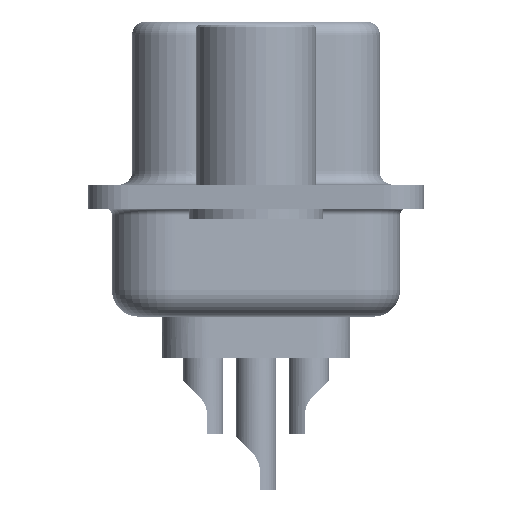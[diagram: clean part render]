
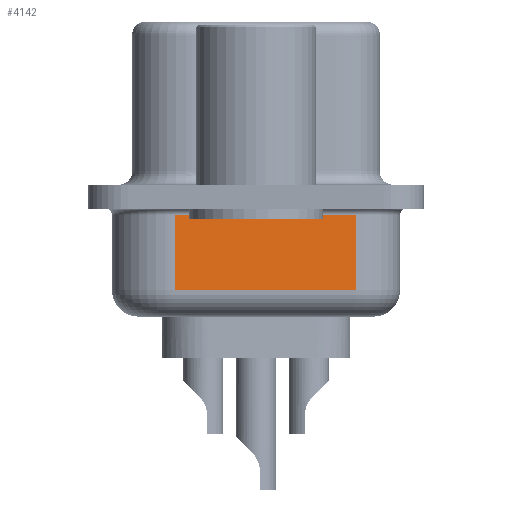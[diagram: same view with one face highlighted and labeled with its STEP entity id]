
A CAD part, left-side view. The second image highlights one B-rep face of the part: STEP entity #4142.
In plain terms, the highlighted planar face has unit normal (-0.985, -0.174, 0).
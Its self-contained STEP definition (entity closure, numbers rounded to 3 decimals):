
#44 = ORIENTED_EDGE ( 'NONE', *, *, #11190, .T. ) ;
#349 = EDGE_LOOP ( 'NONE', ( #19495, #44, #11749, #1574 ) ) ;
#593 = DIRECTION ( 'NONE',  ( 0., 0., 1. ) ) ;
#1041 = LINE ( 'NONE', #5209, #23317 ) ;
#1204 = CARTESIAN_POINT ( 'NONE',  ( 4.199, -3.747, -0.7 ) ) ;
#1379 = LINE ( 'NONE', #17974, #13663 ) ;
#1574 = ORIENTED_EDGE ( 'NONE', *, *, #20124, .T. ) ;
#1625 = FACE_OUTER_BOUND ( 'NONE', #349, .T. ) ;
#1770 = CARTESIAN_POINT ( 'NONE',  ( 3., 3.053, -4.5 ) ) ;
#2224 = VERTEX_POINT ( 'NONE', #1204 ) ;
#2486 = VECTOR ( 'NONE', #16854, 1000. ) ;
#3147 = CARTESIAN_POINT ( 'NONE',  ( 3., 3.053, -3.5 ) ) ;
#4142 = ADVANCED_FACE ( 'NONE', ( #1625 ), #8680, .F. ) ;
#4247 = AXIS2_PLACEMENT_3D ( 'NONE', #1770, #8997, #6689 ) ;
#5209 = CARTESIAN_POINT ( 'NONE',  ( 3., 3.053, -4.5 ) ) ;
#6689 = DIRECTION ( 'NONE',  ( -0.174, 0.985, 0. ) ) ;
#7465 = LINE ( 'NONE', #7762, #2486 ) ;
#7762 = CARTESIAN_POINT ( 'NONE',  ( 4.199, -3.747, -4.5 ) ) ;
#8680 = PLANE ( 'NONE',  #4247 ) ;
#8728 = CARTESIAN_POINT ( 'NONE',  ( 3., 3.053, -0.7 ) ) ;
#8997 = DIRECTION ( 'NONE',  ( 0.985, 0.174, 0. ) ) ;
#11190 = EDGE_CURVE ( 'NONE', #14868, #15572, #1379, .T. ) ;
#11749 = ORIENTED_EDGE ( 'NONE', *, *, #14856, .T. ) ;
#12073 = CARTESIAN_POINT ( 'NONE',  ( 3., 3.053, -0.7 ) ) ;
#13663 = VECTOR ( 'NONE', #17679, 1000. ) ;
#14856 = EDGE_CURVE ( 'NONE', #15572, #2224, #7465, .T. ) ;
#14868 = VERTEX_POINT ( 'NONE', #3147 ) ;
#15572 = VERTEX_POINT ( 'NONE', #24991 ) ;
#16854 = DIRECTION ( 'NONE',  ( 0., 0., 1. ) ) ;
#17679 = DIRECTION ( 'NONE',  ( 0.174, -0.985, 0. ) ) ;
#17690 = VECTOR ( 'NONE', #25213, 1000. ) ;
#17974 = CARTESIAN_POINT ( 'NONE',  ( 3., 3.053, -3.5 ) ) ;
#19495 = ORIENTED_EDGE ( 'NONE', *, *, #25865, .F. ) ;
#20124 = EDGE_CURVE ( 'NONE', #2224, #24507, #22732, .T. ) ;
#22732 = LINE ( 'NONE', #8728, #17690 ) ;
#23317 = VECTOR ( 'NONE', #593, 1000. ) ;
#24507 = VERTEX_POINT ( 'NONE', #12073 ) ;
#24991 = CARTESIAN_POINT ( 'NONE',  ( 4.199, -3.747, -3.5 ) ) ;
#25213 = DIRECTION ( 'NONE',  ( -0.174, 0.985, 0. ) ) ;
#25865 = EDGE_CURVE ( 'NONE', #14868, #24507, #1041, .T. ) ;
